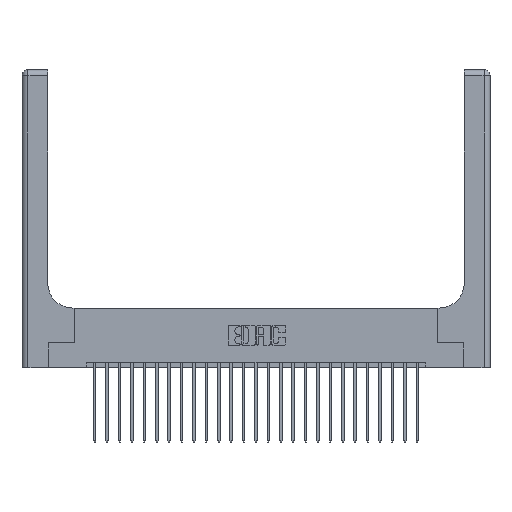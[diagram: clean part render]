
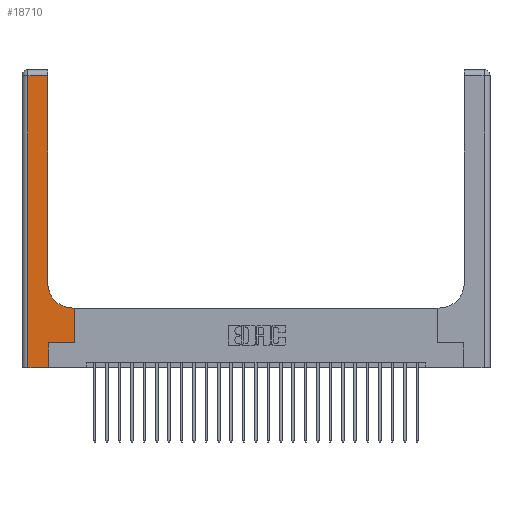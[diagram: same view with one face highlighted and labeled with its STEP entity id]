
A CAD part, top view. The second image highlights one B-rep face of the part: STEP entity #18710.
In plain terms, the highlighted planar face has unit normal (0, 0, 1).
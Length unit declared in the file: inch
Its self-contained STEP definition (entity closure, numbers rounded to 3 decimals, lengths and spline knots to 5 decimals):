
#145 = VECTOR ( 'NONE', #10237, 39.37008 ) ;
#800 = ORIENTED_EDGE ( 'NONE', *, *, #3488, .T. ) ;
#919 = DIRECTION ( 'NONE',  ( 1., 0., 0. ) ) ;
#1328 = CARTESIAN_POINT ( 'NONE',  ( 0., 3., 0.37 ) ) ;
#1336 = DIRECTION ( 'NONE',  ( 0., 1., 0. ) ) ;
#1612 = ORIENTED_EDGE ( 'NONE', *, *, #16864, .T. ) ;
#2185 = VERTEX_POINT ( 'NONE', #16768 ) ;
#2255 = ORIENTED_EDGE ( 'NONE', *, *, #16328, .T. ) ;
#3275 = EDGE_LOOP ( 'NONE', ( #2255, #11212, #13210, #1612, #22933, #16373, #11581, #800, #10595 ) ) ;
#3451 = CARTESIAN_POINT ( 'NONE',  ( 0.265, 0., 0.37 ) ) ;
#3488 = EDGE_CURVE ( 'NONE', #8653, #14824, #20365, .T. ) ;
#3498 = LINE ( 'NONE', #3451, #13450 ) ;
#3915 = EDGE_CURVE ( 'NONE', #7757, #8653, #23369, .T. ) ;
#3921 = DIRECTION ( 'NONE',  ( -1., 0., 0. ) ) ;
#5032 = CARTESIAN_POINT ( 'NONE',  ( 0.26, 2.94, 0.37 ) ) ;
#5066 = VECTOR ( 'NONE', #23798, 39.37008 ) ;
#5220 = LINE ( 'NONE', #20041, #145 ) ;
#6055 = VERTEX_POINT ( 'NONE', #5032 ) ;
#6177 = EDGE_CURVE ( 'NONE', #6055, #13137, #21031, .T. ) ;
#6522 = CARTESIAN_POINT ( 'NONE',  ( 0.26, 3., 0.37 ) ) ;
#7757 = VERTEX_POINT ( 'NONE', #13279 ) ;
#7797 = CARTESIAN_POINT ( 'NONE',  ( 0.26, 0.6, 0.37 ) ) ;
#8653 = VERTEX_POINT ( 'NONE', #14706 ) ;
#8812 = VERTEX_POINT ( 'NONE', #22818 ) ;
#9686 = CARTESIAN_POINT ( 'NONE',  ( 0.51, 0.6, 0.37 ) ) ;
#10237 = DIRECTION ( 'NONE',  ( 0., -1., 0. ) ) ;
#10459 = VECTOR ( 'NONE', #12120, 39.37008 ) ;
#10595 = ORIENTED_EDGE ( 'NONE', *, *, #16147, .T. ) ;
#10703 = DIRECTION ( 'NONE',  ( 0., 0., -1. ) ) ;
#11045 = CARTESIAN_POINT ( 'NONE',  ( 0.528, 0.25, 0.37 ) ) ;
#11212 = ORIENTED_EDGE ( 'NONE', *, *, #6177, .T. ) ;
#11581 = ORIENTED_EDGE ( 'NONE', *, *, #3915, .T. ) ;
#11722 = CIRCLE ( 'NONE', #18779, 0.25 ) ;
#11816 = DIRECTION ( 'NONE',  ( 1., 0., 0. ) ) ;
#12120 = DIRECTION ( 'NONE',  ( 1., 0., 0. ) ) ;
#12878 = VECTOR ( 'NONE', #1336, 39.37008 ) ;
#13137 = VERTEX_POINT ( 'NONE', #23325 ) ;
#13182 = CARTESIAN_POINT ( 'NONE',  ( 0.265, 0.25, 0.37 ) ) ;
#13210 = ORIENTED_EDGE ( 'NONE', *, *, #18641, .T. ) ;
#13279 = CARTESIAN_POINT ( 'NONE',  ( 0.528, 0.25, 0.37 ) ) ;
#13410 = EDGE_CURVE ( 'NONE', #21442, #7757, #19354, .T. ) ;
#13450 = VECTOR ( 'NONE', #18596, 39.37008 ) ;
#13986 = CARTESIAN_POINT ( 'NONE',  ( 0., 0., 0.37 ) ) ;
#14508 = AXIS2_PLACEMENT_3D ( 'NONE', #1328, #10703, #24390 ) ;
#14706 = CARTESIAN_POINT ( 'NONE',  ( 0.528, 0.6, 0.37 ) ) ;
#14824 = VERTEX_POINT ( 'NONE', #9686 ) ;
#14976 = LINE ( 'NONE', #13986, #10459 ) ;
#15289 = VECTOR ( 'NONE', #3921, 39.37008 ) ;
#16147 = EDGE_CURVE ( 'NONE', #14824, #8812, #11722, .T. ) ;
#16328 = EDGE_CURVE ( 'NONE', #8812, #6055, #17111, .T. ) ;
#16373 = ORIENTED_EDGE ( 'NONE', *, *, #13410, .T. ) ;
#16768 = CARTESIAN_POINT ( 'NONE',  ( 0.265, 0., 0.37 ) ) ;
#16864 = EDGE_CURVE ( 'NONE', #21359, #2185, #14976, .T. ) ;
#16876 = CARTESIAN_POINT ( 'NONE',  ( 0., 2.94, 0.37 ) ) ;
#17111 = LINE ( 'NONE', #6522, #5066 ) ;
#18550 = CARTESIAN_POINT ( 'NONE',  ( 0.06, 0., 0.37 ) ) ;
#18596 = DIRECTION ( 'NONE',  ( 0., 1., 0. ) ) ;
#18641 = EDGE_CURVE ( 'NONE', #13137, #21359, #5220, .T. ) ;
#18710 = ADVANCED_FACE ( 'NONE', ( #24452 ), #24057, .F. ) ;
#18779 = AXIS2_PLACEMENT_3D ( 'NONE', #19289, #23306, #11816 ) ;
#18821 = DIRECTION ( 'NONE',  ( -1., 0., 0. ) ) ;
#19289 = CARTESIAN_POINT ( 'NONE',  ( 0.51, 0.85, 0.37 ) ) ;
#19354 = LINE ( 'NONE', #23812, #20876 ) ;
#20041 = CARTESIAN_POINT ( 'NONE',  ( 0.06, 3., 0.37 ) ) ;
#20365 = LINE ( 'NONE', #7797, #15289 ) ;
#20876 = VECTOR ( 'NONE', #919, 39.37008 ) ;
#21031 = LINE ( 'NONE', #16876, #21354 ) ;
#21354 = VECTOR ( 'NONE', #18821, 39.37008 ) ;
#21359 = VERTEX_POINT ( 'NONE', #18550 ) ;
#21442 = VERTEX_POINT ( 'NONE', #13182 ) ;
#22818 = CARTESIAN_POINT ( 'NONE',  ( 0.26, 0.85, 0.37 ) ) ;
#22933 = ORIENTED_EDGE ( 'NONE', *, *, #23956, .T. ) ;
#23306 = DIRECTION ( 'NONE',  ( 0., 0., -1. ) ) ;
#23325 = CARTESIAN_POINT ( 'NONE',  ( 0.06, 2.94, 0.37 ) ) ;
#23369 = LINE ( 'NONE', #11045, #12878 ) ;
#23798 = DIRECTION ( 'NONE',  ( 0., 1., 0. ) ) ;
#23812 = CARTESIAN_POINT ( 'NONE',  ( 0.265, 0.25, 0.37 ) ) ;
#23956 = EDGE_CURVE ( 'NONE', #2185, #21442, #3498, .T. ) ;
#24057 = PLANE ( 'NONE',  #14508 ) ;
#24390 = DIRECTION ( 'NONE',  ( -1., 0., 0. ) ) ;
#24452 = FACE_OUTER_BOUND ( 'NONE', #3275, .T. ) ;
